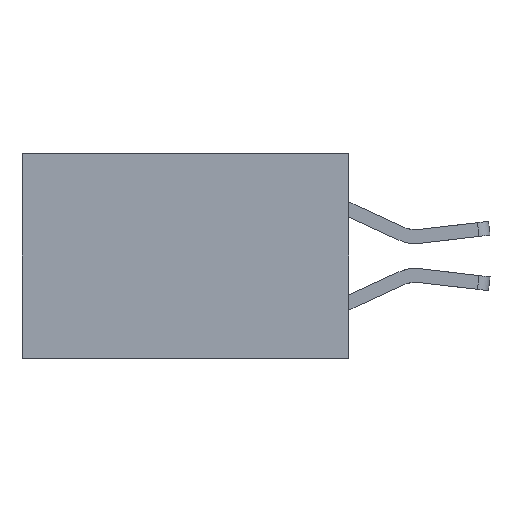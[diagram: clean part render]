
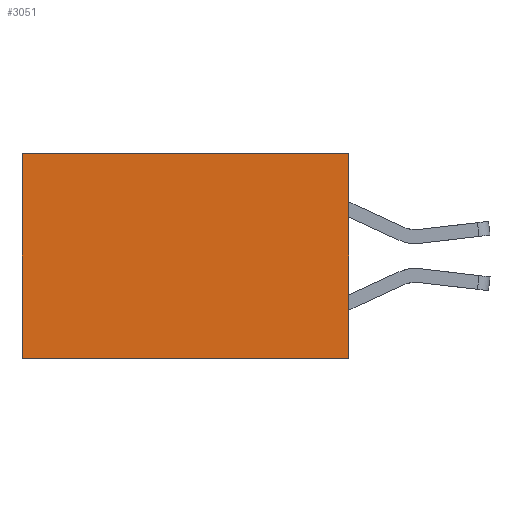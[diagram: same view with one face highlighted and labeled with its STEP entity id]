
A CAD part, left-side view. The second image highlights one B-rep face of the part: STEP entity #3051.
In plain terms, the highlighted planar face has unit normal (-1, 0, 0).
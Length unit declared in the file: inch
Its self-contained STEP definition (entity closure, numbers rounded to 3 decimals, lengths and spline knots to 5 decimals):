
#574 = VECTOR ( 'NONE', #8491, 39.37008 ) ;
#690 = DIRECTION ( 'NONE',  ( 0., 0., -1. ) ) ;
#1224 = ORIENTED_EDGE ( 'NONE', *, *, #3598, .F. ) ;
#1262 = CARTESIAN_POINT ( 'NONE',  ( 0.277, 0., -0.37 ) ) ;
#1601 = DIRECTION ( 'NONE',  ( 0., 0., -1. ) ) ;
#1620 = DIRECTION ( 'NONE',  ( 1., 0., 0. ) ) ;
#1633 = CARTESIAN_POINT ( 'NONE',  ( 0.277, 0., -0.37 ) ) ;
#1743 = PLANE ( 'NONE',  #4960 ) ;
#1807 = EDGE_LOOP ( 'NONE', ( #8340, #1224, #3164, #4993 ) ) ;
#1961 = FACE_OUTER_BOUND ( 'NONE', #1807, .T. ) ;
#2490 = VERTEX_POINT ( 'NONE', #2967 ) ;
#2528 = VECTOR ( 'NONE', #690, 39.37008 ) ;
#2656 = VERTEX_POINT ( 'NONE', #4585 ) ;
#2731 = VECTOR ( 'NONE', #8006, 39.37008 ) ;
#2967 = CARTESIAN_POINT ( 'NONE',  ( 0.277, 0., -0.37 ) ) ;
#3051 = ADVANCED_FACE ( 'NONE', ( #1961 ), #1743, .F. ) ;
#3164 = ORIENTED_EDGE ( 'NONE', *, *, #3216, .F. ) ;
#3216 = EDGE_CURVE ( 'NONE', #2656, #2490, #7761, .T. ) ;
#3489 = VERTEX_POINT ( 'NONE', #7086 ) ;
#3598 = EDGE_CURVE ( 'NONE', #2490, #6586, #4816, .T. ) ;
#4501 = CARTESIAN_POINT ( 'NONE',  ( 0.277, 0.59, -0.37 ) ) ;
#4538 = EDGE_CURVE ( 'NONE', #2656, #3489, #8159, .T. ) ;
#4585 = CARTESIAN_POINT ( 'NONE',  ( 0.277, 0., 0. ) ) ;
#4816 = LINE ( 'NONE', #8423, #574 ) ;
#4960 = AXIS2_PLACEMENT_3D ( 'NONE', #1633, #1620, #1601 ) ;
#4993 = ORIENTED_EDGE ( 'NONE', *, *, #4538, .T. ) ;
#4995 = VECTOR ( 'NONE', #7053, 39.37008 ) ;
#5990 = EDGE_CURVE ( 'NONE', #3489, #6586, #6596, .T. ) ;
#6586 = VERTEX_POINT ( 'NONE', #4501 ) ;
#6596 = LINE ( 'NONE', #7052, #4995 ) ;
#7052 = CARTESIAN_POINT ( 'NONE',  ( 0.277, 0.59, -0.37 ) ) ;
#7053 = DIRECTION ( 'NONE',  ( 0., 0., -1. ) ) ;
#7086 = CARTESIAN_POINT ( 'NONE',  ( 0.277, 0.59, 0. ) ) ;
#7761 = LINE ( 'NONE', #1262, #2528 ) ;
#8006 = DIRECTION ( 'NONE',  ( 0., 1., 0. ) ) ;
#8159 = LINE ( 'NONE', #8294, #2731 ) ;
#8294 = CARTESIAN_POINT ( 'NONE',  ( 0.277, 0., 0. ) ) ;
#8340 = ORIENTED_EDGE ( 'NONE', *, *, #5990, .T. ) ;
#8423 = CARTESIAN_POINT ( 'NONE',  ( 0.277, 0., -0.37 ) ) ;
#8491 = DIRECTION ( 'NONE',  ( 0., 1., 0. ) ) ;
